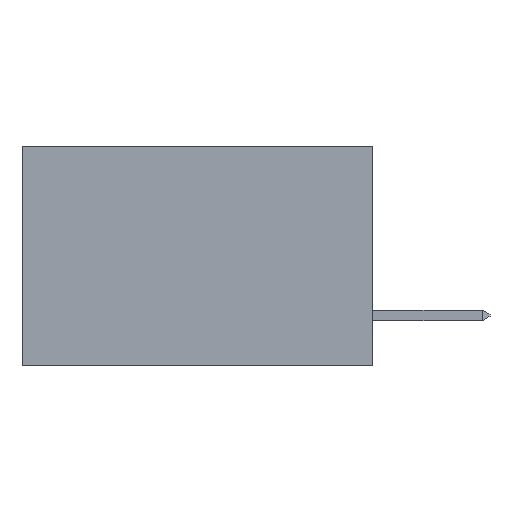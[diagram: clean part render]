
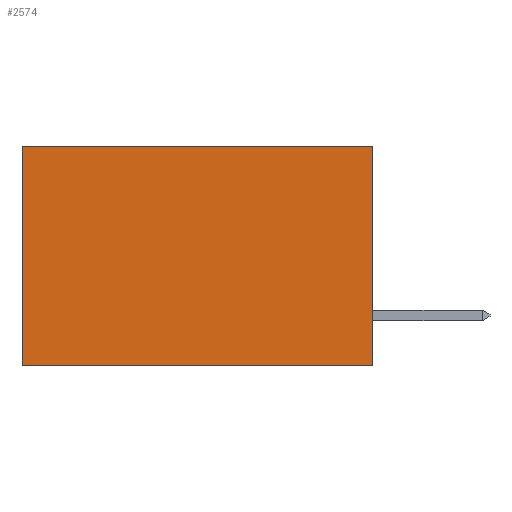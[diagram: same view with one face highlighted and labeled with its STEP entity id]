
A CAD part, left-side view. The second image highlights one B-rep face of the part: STEP entity #2574.
In plain terms, the highlighted planar face has unit normal (-1, 0, 0).
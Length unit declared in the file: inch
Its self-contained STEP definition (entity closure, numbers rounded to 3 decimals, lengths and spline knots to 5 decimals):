
#63 = CARTESIAN_POINT ( 'NONE',  ( 0.277, 0., -0.37 ) ) ;
#553 = VERTEX_POINT ( 'NONE', #6183 ) ;
#672 = CARTESIAN_POINT ( 'NONE',  ( 0.277, 0., -0.37 ) ) ;
#757 = EDGE_CURVE ( 'NONE', #553, #1343, #7662, .T. ) ;
#798 = LINE ( 'NONE', #4960, #8737 ) ;
#840 = PLANE ( 'NONE',  #4251 ) ;
#1112 = DIRECTION ( 'NONE',  ( 0., 0., -1. ) ) ;
#1153 = DIRECTION ( 'NONE',  ( 1., 0., 0. ) ) ;
#1343 = VERTEX_POINT ( 'NONE', #7267 ) ;
#1879 = DIRECTION ( 'NONE',  ( 0., 0., -1. ) ) ;
#1897 = CARTESIAN_POINT ( 'NONE',  ( 0.277, 0., -0.37 ) ) ;
#1923 = DIRECTION ( 'NONE',  ( 0., 1., 0. ) ) ;
#2280 = LINE ( 'NONE', #672, #6593 ) ;
#2574 = ADVANCED_FACE ( 'NONE', ( #5277 ), #840, .F. ) ;
#2652 = EDGE_CURVE ( 'NONE', #3025, #553, #2280, .T. ) ;
#3025 = VERTEX_POINT ( 'NONE', #8548 ) ;
#3220 = LINE ( 'NONE', #3614, #6995 ) ;
#3266 = ORIENTED_EDGE ( 'NONE', *, *, #6984, .T. ) ;
#3333 = EDGE_LOOP ( 'NONE', ( #3266, #7279, #3510, #7503 ) ) ;
#3343 = VERTEX_POINT ( 'NONE', #7609 ) ;
#3510 = ORIENTED_EDGE ( 'NONE', *, *, #2652, .F. ) ;
#3583 = DIRECTION ( 'NONE',  ( 0., 1., 0. ) ) ;
#3614 = CARTESIAN_POINT ( 'NONE',  ( 0.277, 0., 0. ) ) ;
#4251 = AXIS2_PLACEMENT_3D ( 'NONE', #63, #1153, #1112 ) ;
#4960 = CARTESIAN_POINT ( 'NONE',  ( 0.277, 0.59, -0.37 ) ) ;
#5024 = DIRECTION ( 'NONE',  ( 0., 0., -1. ) ) ;
#5150 = EDGE_CURVE ( 'NONE', #3025, #3343, #3220, .T. ) ;
#5277 = FACE_OUTER_BOUND ( 'NONE', #3333, .T. ) ;
#6183 = CARTESIAN_POINT ( 'NONE',  ( 0.277, 0., -0.37 ) ) ;
#6593 = VECTOR ( 'NONE', #1879, 39.37008 ) ;
#6984 = EDGE_CURVE ( 'NONE', #3343, #1343, #798, .T. ) ;
#6995 = VECTOR ( 'NONE', #3583, 39.37008 ) ;
#7267 = CARTESIAN_POINT ( 'NONE',  ( 0.277, 0.59, -0.37 ) ) ;
#7279 = ORIENTED_EDGE ( 'NONE', *, *, #757, .F. ) ;
#7503 = ORIENTED_EDGE ( 'NONE', *, *, #5150, .T. ) ;
#7609 = CARTESIAN_POINT ( 'NONE',  ( 0.277, 0.59, 0. ) ) ;
#7662 = LINE ( 'NONE', #1897, #9781 ) ;
#8548 = CARTESIAN_POINT ( 'NONE',  ( 0.277, 0., 0. ) ) ;
#8737 = VECTOR ( 'NONE', #5024, 39.37008 ) ;
#9781 = VECTOR ( 'NONE', #1923, 39.37008 ) ;
